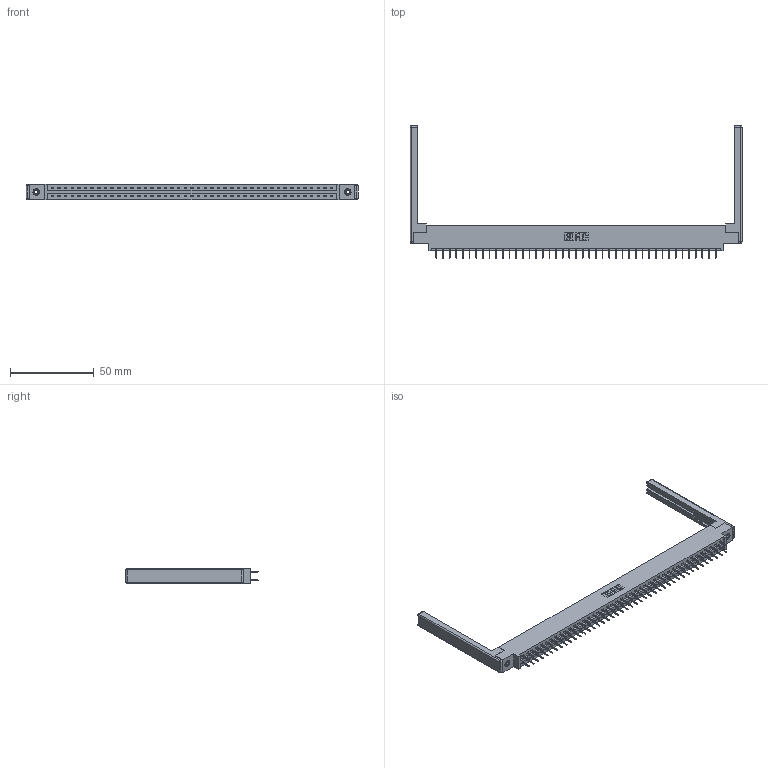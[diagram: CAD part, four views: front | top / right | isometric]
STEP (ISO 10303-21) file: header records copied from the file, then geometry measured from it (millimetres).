
FILE_DESCRIPTION (( 'STEP AP203' ), '1' );
FILE_NAME ('337-086-524-868.STEP', '2019-10-15T18:48:07', ( '' ), ( '' ), 'SwSTEP 2.0', 'SolidWorks 2016', '' );
FILE_SCHEMA (( 'CONFIG_CONTROL_DESIGN' ));
Length unit declared in the file: inch
Products named in the file (5): 345-250-001_345-250-001-102; 337 Part_0.170 Offset - 0.156 Dia-TI; 307-220-068; 337-086-524-868; 345-292-001_345-293-124
Assembly tree (91 placements, depth 2):
  337-086-524-868
    337 Part_0.170 Offset - 0.156 Dia-TI
    345-292-001_345-293-124  x86
    345-250-001_345-250-001-102  x2
    307-220-068  x2
Bounding box: 197.82 x 78.75 x 9.4 mm (x, y, z)
Volume: 24997.8 mm3; surface area: 27051.9 mm2
Topology: 91 solids, 91 shells, 5260 faces, 14903 edges, 9570 vertices
Faces by surface type: plane 3946, cylinder 1290, cone 12, sphere 8, torus 4
Entity records: 36176 total; most frequent: CARTESIAN_POINT 6059, ORIENTED_EDGE 5984, DIRECTION 5222, EDGE_CURVE 2992, LINE 2818, VECTOR 2818, VERTEX_POINT 1982, AXIS2_PLACEMENT_3D 1202
